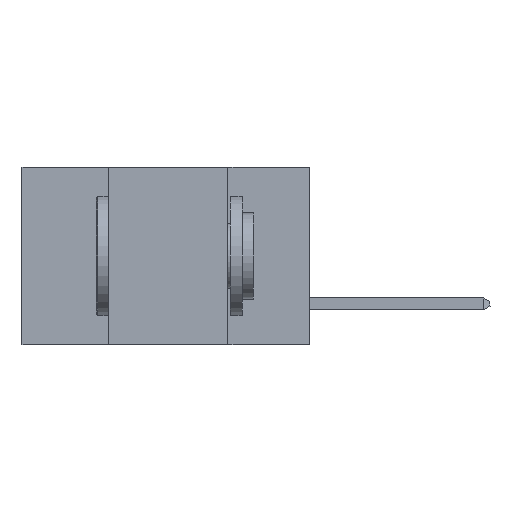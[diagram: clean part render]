
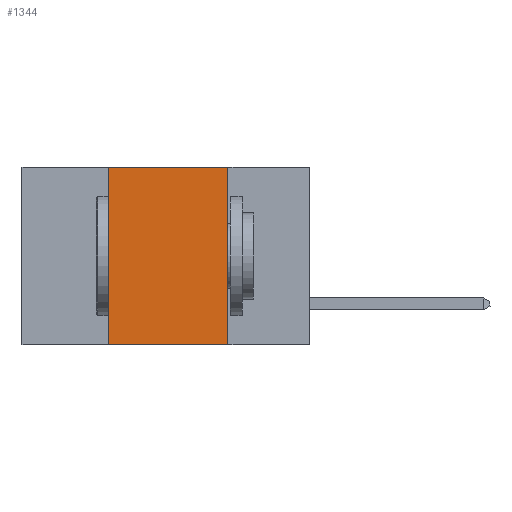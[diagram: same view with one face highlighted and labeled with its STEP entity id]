
A CAD part, left-side view. The second image highlights one B-rep face of the part: STEP entity #1344.
In plain terms, the highlighted planar face has unit normal (-1, 0, 0).
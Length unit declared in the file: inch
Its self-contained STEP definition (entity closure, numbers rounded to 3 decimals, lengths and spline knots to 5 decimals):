
#411 = EDGE_CURVE ( 'NONE', #14518, #9729, #5523, .T. ) ;
#481 = CARTESIAN_POINT ( 'NONE',  ( 0., 0.42, -0.37 ) ) ;
#992 = CARTESIAN_POINT ( 'NONE',  ( 0., 0.17, 0. ) ) ;
#1344 = ADVANCED_FACE ( 'NONE', ( #6341 ), #10813, .F. ) ;
#2474 = ORIENTED_EDGE ( 'NONE', *, *, #5417, .F. ) ;
#2769 = ORIENTED_EDGE ( 'NONE', *, *, #411, .F. ) ;
#3216 = CARTESIAN_POINT ( 'NONE',  ( 0., 0.42, 0. ) ) ;
#3638 = VERTEX_POINT ( 'NONE', #992 ) ;
#4826 = DIRECTION ( 'NONE',  ( 0., -1., 0. ) ) ;
#5417 = EDGE_CURVE ( 'NONE', #9729, #3638, #16198, .T. ) ;
#5523 = LINE ( 'NONE', #3216, #12247 ) ;
#5783 = CARTESIAN_POINT ( 'NONE',  ( 0., 0.6, 0. ) ) ;
#6064 = EDGE_LOOP ( 'NONE', ( #13131, #2474, #2769, #7275 ) ) ;
#6341 = FACE_OUTER_BOUND ( 'NONE', #6064, .T. ) ;
#7275 = ORIENTED_EDGE ( 'NONE', *, *, #12774, .T. ) ;
#7346 = CARTESIAN_POINT ( 'NONE',  ( 0., 0.17, -0.37 ) ) ;
#7778 = VECTOR ( 'NONE', #4826, 39.37008 ) ;
#8334 = DIRECTION ( 'NONE',  ( 0., 0., -1. ) ) ;
#8500 = DIRECTION ( 'NONE',  ( 0., 0., -1. ) ) ;
#8659 = CARTESIAN_POINT ( 'NONE',  ( 0., 0.17, 0. ) ) ;
#8664 = CARTESIAN_POINT ( 'NONE',  ( 0., 0.6, 0. ) ) ;
#9729 = VERTEX_POINT ( 'NONE', #16133 ) ;
#10069 = VECTOR ( 'NONE', #15655, 39.37008 ) ;
#10495 = EDGE_CURVE ( 'NONE', #3638, #12190, #12900, .T. ) ;
#10813 = PLANE ( 'NONE',  #11554 ) ;
#10925 = DIRECTION ( 'NONE',  ( 1., 0., 0. ) ) ;
#11554 = AXIS2_PLACEMENT_3D ( 'NONE', #5783, #10925, #8334 ) ;
#11963 = CARTESIAN_POINT ( 'NONE',  ( 0., 0.6, -0.37 ) ) ;
#12190 = VERTEX_POINT ( 'NONE', #7346 ) ;
#12247 = VECTOR ( 'NONE', #13117, 39.37008 ) ;
#12774 = EDGE_CURVE ( 'NONE', #14518, #12190, #13615, .T. ) ;
#12900 = LINE ( 'NONE', #8659, #13683 ) ;
#13117 = DIRECTION ( 'NONE',  ( 0., 0., 1. ) ) ;
#13131 = ORIENTED_EDGE ( 'NONE', *, *, #10495, .F. ) ;
#13615 = LINE ( 'NONE', #11963, #10069 ) ;
#13683 = VECTOR ( 'NONE', #8500, 39.37008 ) ;
#14518 = VERTEX_POINT ( 'NONE', #481 ) ;
#15655 = DIRECTION ( 'NONE',  ( 0., -1., 0. ) ) ;
#16133 = CARTESIAN_POINT ( 'NONE',  ( 0., 0.42, 0. ) ) ;
#16198 = LINE ( 'NONE', #8664, #7778 ) ;
